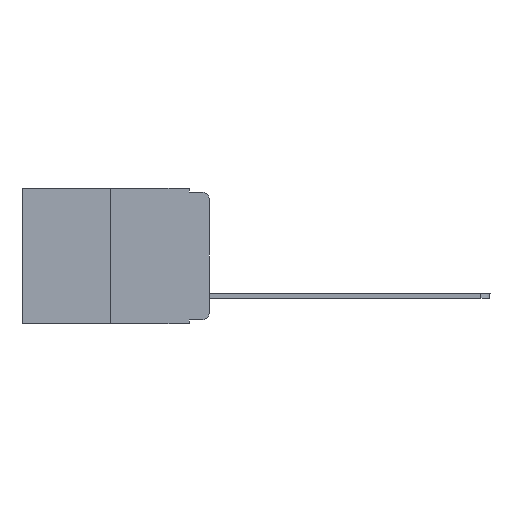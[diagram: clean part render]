
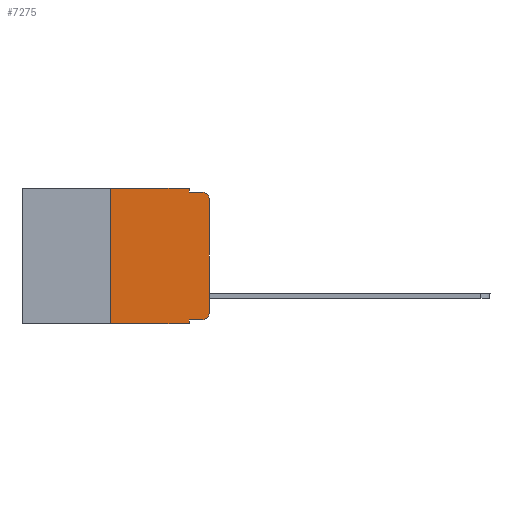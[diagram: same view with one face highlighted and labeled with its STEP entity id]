
A CAD part, left-side view. The second image highlights one B-rep face of the part: STEP entity #7275.
In plain terms, the highlighted planar face has unit normal (-1, 0, 0).
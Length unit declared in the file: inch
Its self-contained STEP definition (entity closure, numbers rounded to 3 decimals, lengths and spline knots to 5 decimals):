
#17 = LINE ( 'NONE', #6806, #3522 ) ;
#96 = CARTESIAN_POINT ( 'NONE',  ( 0., 0.02, -0.333 ) ) ;
#518 = ORIENTED_EDGE ( 'NONE', *, *, #2741, .F. ) ;
#1815 = CARTESIAN_POINT ( 'NONE',  ( 0., 0.25, -0.343 ) ) ;
#2549 = CARTESIAN_POINT ( 'NONE',  ( 0., 0.051, -0.01 ) ) ;
#2595 = VERTEX_POINT ( 'NONE', #3559 ) ;
#2611 = DIRECTION ( 'NONE',  ( 0., 0., 1. ) ) ;
#2715 = LINE ( 'NONE', #7389, #12261 ) ;
#2741 = EDGE_CURVE ( 'NONE', #2595, #14124, #7547, .T. ) ;
#3125 = EDGE_CURVE ( 'NONE', #3443, #21721, #2715, .T. ) ;
#3443 = VERTEX_POINT ( 'NONE', #1815 ) ;
#3522 = VECTOR ( 'NONE', #13595, 39.37008 ) ;
#3559 = CARTESIAN_POINT ( 'NONE',  ( 0., 0.051, 0. ) ) ;
#3630 = DIRECTION ( 'NONE',  ( 0., 0., -1. ) ) ;
#4099 = ORIENTED_EDGE ( 'NONE', *, *, #19786, .T. ) ;
#4200 = LINE ( 'NONE', #9434, #18227 ) ;
#5171 = EDGE_CURVE ( 'NONE', #14124, #17826, #7342, .T. ) ;
#5417 = PLANE ( 'NONE',  #11473 ) ;
#5600 = VERTEX_POINT ( 'NONE', #17442 ) ;
#5769 = CARTESIAN_POINT ( 'NONE',  ( 0., 0.051, 0. ) ) ;
#5958 = LINE ( 'NONE', #7623, #21809 ) ;
#6729 = LINE ( 'NONE', #18634, #19574 ) ;
#6806 = CARTESIAN_POINT ( 'NONE',  ( 0., 0.473, -0.343 ) ) ;
#6920 = VERTEX_POINT ( 'NONE', #17785 ) ;
#7045 = ORIENTED_EDGE ( 'NONE', *, *, #20034, .T. ) ;
#7275 = ADVANCED_FACE ( 'NONE', ( #9091 ), #5417, .F. ) ;
#7342 = LINE ( 'NONE', #2549, #13124 ) ;
#7389 = CARTESIAN_POINT ( 'NONE',  ( 0., 0.25, 0. ) ) ;
#7547 = LINE ( 'NONE', #5769, #16856 ) ;
#7623 = CARTESIAN_POINT ( 'NONE',  ( 0., 0., 0. ) ) ;
#7713 = ORIENTED_EDGE ( 'NONE', *, *, #21481, .F. ) ;
#7762 = DIRECTION ( 'NONE',  ( 0., 0., -1. ) ) ;
#8597 = CARTESIAN_POINT ( 'NONE',  ( 0., 0.051, -0.343 ) ) ;
#8731 = DIRECTION ( 'NONE',  ( -1., 0., 0. ) ) ;
#9091 = FACE_OUTER_BOUND ( 'NONE', #11716, .T. ) ;
#9434 = CARTESIAN_POINT ( 'NONE',  ( 0., 0.051, 0. ) ) ;
#10316 = DIRECTION ( 'NONE',  ( 1., 0., 0. ) ) ;
#10385 = EDGE_CURVE ( 'NONE', #5600, #19938, #5958, .T. ) ;
#11047 = DIRECTION ( 'NONE',  ( -1., 0., 0. ) ) ;
#11271 = DIRECTION ( 'NONE',  ( 0., 0., -1. ) ) ;
#11473 = AXIS2_PLACEMENT_3D ( 'NONE', #15873, #10316, #3630 ) ;
#11716 = EDGE_LOOP ( 'NONE', ( #20874, #4099, #20962, #518, #7713, #21098, #7045, #20304, #21278, #15740 ) ) ;
#12261 = VECTOR ( 'NONE', #17517, 39.37008 ) ;
#12778 = CIRCLE ( 'NONE', #18447, 0.02 ) ;
#13124 = VECTOR ( 'NONE', #14133, 39.37008 ) ;
#13595 = DIRECTION ( 'NONE',  ( 0., -1., 0. ) ) ;
#13796 = EDGE_CURVE ( 'NONE', #6920, #21906, #18469, .T. ) ;
#14124 = VERTEX_POINT ( 'NONE', #17787 ) ;
#14133 = DIRECTION ( 'NONE',  ( 0., -1., 0. ) ) ;
#14273 = CARTESIAN_POINT ( 'NONE',  ( 0., 0.02, -0.03 ) ) ;
#14550 = CIRCLE ( 'NONE', #21680, 0.02 ) ;
#14918 = CARTESIAN_POINT ( 'NONE',  ( 0., 0.25, 0. ) ) ;
#15512 = DIRECTION ( 'NONE',  ( 0., 0., -1. ) ) ;
#15740 = ORIENTED_EDGE ( 'NONE', *, *, #19899, .T. ) ;
#15873 = CARTESIAN_POINT ( 'NONE',  ( 0., 0.473, 0. ) ) ;
#16011 = DIRECTION ( 'NONE',  ( 0., 0., -1. ) ) ;
#16045 = CARTESIAN_POINT ( 'NONE',  ( 0., 0.02, -0.313 ) ) ;
#16576 = DIRECTION ( 'NONE',  ( 0., -1., 0. ) ) ;
#16620 = VERTEX_POINT ( 'NONE', #8597 ) ;
#16707 = CARTESIAN_POINT ( 'NONE',  ( 0., 0.02, -0.01 ) ) ;
#16856 = VECTOR ( 'NONE', #16011, 39.37008 ) ;
#17442 = CARTESIAN_POINT ( 'NONE',  ( 0., 0., -0.313 ) ) ;
#17517 = DIRECTION ( 'NONE',  ( 0., 0., 1. ) ) ;
#17785 = CARTESIAN_POINT ( 'NONE',  ( 0., 0.051, -0.333 ) ) ;
#17787 = CARTESIAN_POINT ( 'NONE',  ( 0., 0.051, -0.01 ) ) ;
#17826 = VERTEX_POINT ( 'NONE', #16707 ) ;
#18227 = VECTOR ( 'NONE', #7762, 39.37008 ) ;
#18447 = AXIS2_PLACEMENT_3D ( 'NONE', #16045, #11047, #11271 ) ;
#18469 = LINE ( 'NONE', #20040, #21511 ) ;
#18599 = CARTESIAN_POINT ( 'NONE',  ( 0., 0., -0.03 ) ) ;
#18634 = CARTESIAN_POINT ( 'NONE',  ( 0., 0.473, 0. ) ) ;
#19574 = VECTOR ( 'NONE', #20753, 39.37008 ) ;
#19786 = EDGE_CURVE ( 'NONE', #19938, #17826, #14550, .T. ) ;
#19899 = EDGE_CURVE ( 'NONE', #21906, #5600, #12778, .T. ) ;
#19938 = VERTEX_POINT ( 'NONE', #18599 ) ;
#20034 = EDGE_CURVE ( 'NONE', #3443, #16620, #17, .T. ) ;
#20040 = CARTESIAN_POINT ( 'NONE',  ( 0., 0.051, -0.333 ) ) ;
#20304 = ORIENTED_EDGE ( 'NONE', *, *, #21986, .F. ) ;
#20753 = DIRECTION ( 'NONE',  ( 0., -1., 0. ) ) ;
#20874 = ORIENTED_EDGE ( 'NONE', *, *, #10385, .T. ) ;
#20962 = ORIENTED_EDGE ( 'NONE', *, *, #5171, .F. ) ;
#21098 = ORIENTED_EDGE ( 'NONE', *, *, #3125, .F. ) ;
#21278 = ORIENTED_EDGE ( 'NONE', *, *, #13796, .T. ) ;
#21481 = EDGE_CURVE ( 'NONE', #21721, #2595, #6729, .T. ) ;
#21511 = VECTOR ( 'NONE', #16576, 39.37008 ) ;
#21680 = AXIS2_PLACEMENT_3D ( 'NONE', #14273, #8731, #15512 ) ;
#21721 = VERTEX_POINT ( 'NONE', #14918 ) ;
#21809 = VECTOR ( 'NONE', #2611, 39.37008 ) ;
#21906 = VERTEX_POINT ( 'NONE', #96 ) ;
#21986 = EDGE_CURVE ( 'NONE', #6920, #16620, #4200, .T. ) ;
